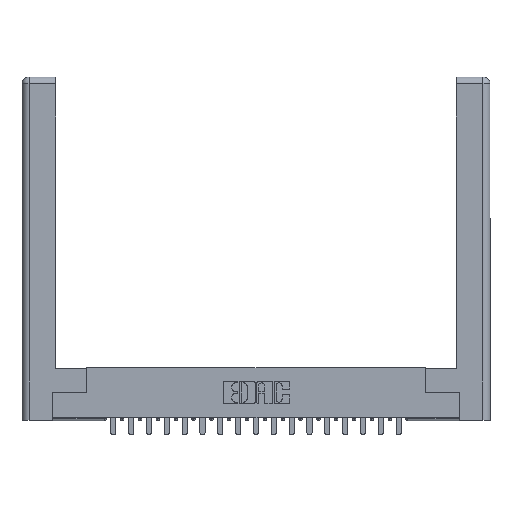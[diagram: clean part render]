
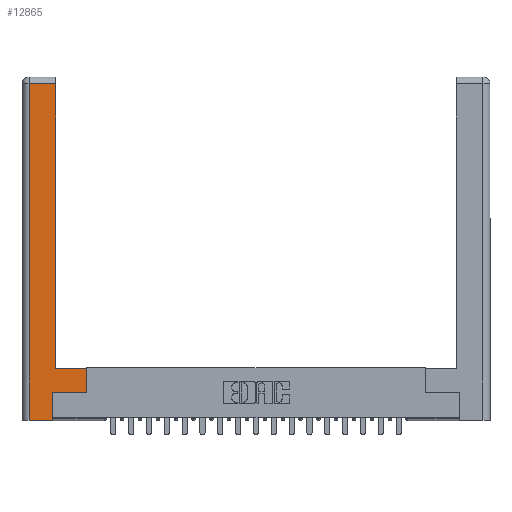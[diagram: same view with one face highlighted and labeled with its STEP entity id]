
A CAD part, top view. The second image highlights one B-rep face of the part: STEP entity #12865.
In plain terms, the highlighted planar face has unit normal (0, 0, 1).
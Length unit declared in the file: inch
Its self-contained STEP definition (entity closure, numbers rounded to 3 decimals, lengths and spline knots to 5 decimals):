
#217 = VECTOR ( 'NONE', #2579, 39.37008 ) ;
#251 = VERTEX_POINT ( 'NONE', #19789 ) ;
#571 = CARTESIAN_POINT ( 'NONE',  ( 0.295, 0.45, 0. ) ) ;
#2059 = EDGE_CURVE ( 'NONE', #21015, #13240, #12408, .T. ) ;
#2579 = DIRECTION ( 'NONE',  ( 1., 0., 0. ) ) ;
#3246 = DIRECTION ( 'NONE',  ( -1., 0., 0. ) ) ;
#3334 = PLANE ( 'NONE',  #18562 ) ;
#3410 = VECTOR ( 'NONE', #20492, 39.37008 ) ;
#3704 = ORIENTED_EDGE ( 'NONE', *, *, #23173, .T. ) ;
#3759 = DIRECTION ( 'NONE',  ( 0., -1., 0. ) ) ;
#4074 = CARTESIAN_POINT ( 'NONE',  ( 0.0615, 0., 0. ) ) ;
#4550 = ORIENTED_EDGE ( 'NONE', *, *, #2059, .T. ) ;
#4718 = CARTESIAN_POINT ( 'NONE',  ( 0.265, 0.245, 0. ) ) ;
#5852 = LINE ( 'NONE', #7973, #15176 ) ;
#6059 = DIRECTION ( 'NONE',  ( -1., 0., 0. ) ) ;
#6179 = CARTESIAN_POINT ( 'NONE',  ( 0.565, 0.45, 0. ) ) ;
#6319 = DIRECTION ( 'NONE',  ( 0., 1., 0. ) ) ;
#6332 = DIRECTION ( 'NONE',  ( -1., 0., 0. ) ) ;
#6421 = FACE_OUTER_BOUND ( 'NONE', #18535, .T. ) ;
#7001 = VERTEX_POINT ( 'NONE', #9324 ) ;
#7973 = CARTESIAN_POINT ( 'NONE',  ( 0.295, 0.45, 0. ) ) ;
#8054 = EDGE_CURVE ( 'NONE', #251, #20877, #14754, .T. ) ;
#8365 = ORIENTED_EDGE ( 'NONE', *, *, #20560, .T. ) ;
#8759 = CARTESIAN_POINT ( 'NONE',  ( 0., 0., 0. ) ) ;
#8888 = CARTESIAN_POINT ( 'NONE',  ( 0.565, 0.245, 0. ) ) ;
#9078 = DIRECTION ( 'NONE',  ( 0., 1., 0. ) ) ;
#9324 = CARTESIAN_POINT ( 'NONE',  ( 0.265, 0., 0. ) ) ;
#9907 = LINE ( 'NONE', #23638, #19163 ) ;
#9926 = EDGE_CURVE ( 'NONE', #14720, #12244, #15286, .T. ) ;
#10376 = ORIENTED_EDGE ( 'NONE', *, *, #16593, .T. ) ;
#10413 = ORIENTED_EDGE ( 'NONE', *, *, #12035, .T. ) ;
#10781 = DIRECTION ( 'NONE',  ( 1., 0., 0. ) ) ;
#12035 = EDGE_CURVE ( 'NONE', #12323, #251, #16365, .T. ) ;
#12057 = CARTESIAN_POINT ( 'NONE',  ( 0.0615, 0., 0. ) ) ;
#12240 = ORIENTED_EDGE ( 'NONE', *, *, #18211, .T. ) ;
#12244 = VERTEX_POINT ( 'NONE', #12057 ) ;
#12323 = VERTEX_POINT ( 'NONE', #4718 ) ;
#12408 = LINE ( 'NONE', #17141, #20802 ) ;
#12722 = CARTESIAN_POINT ( 'NONE',  ( 0.0615, 2.94, 0. ) ) ;
#12865 = ADVANCED_FACE ( 'NONE', ( #6421 ), #3334, .F. ) ;
#12906 = VECTOR ( 'NONE', #3759, 39.37008 ) ;
#13240 = VERTEX_POINT ( 'NONE', #16415 ) ;
#14352 = DIRECTION ( 'NONE',  ( 0., 0., -1. ) ) ;
#14720 = VERTEX_POINT ( 'NONE', #12722 ) ;
#14754 = LINE ( 'NONE', #20574, #3410 ) ;
#15176 = VECTOR ( 'NONE', #6332, 39.37008 ) ;
#15286 = LINE ( 'NONE', #4074, #12906 ) ;
#16306 = ORIENTED_EDGE ( 'NONE', *, *, #8054, .T. ) ;
#16365 = LINE ( 'NONE', #8888, #20684 ) ;
#16415 = CARTESIAN_POINT ( 'NONE',  ( 0.295, 2.94, 0. ) ) ;
#16593 = EDGE_CURVE ( 'NONE', #12244, #7001, #18201, .T. ) ;
#17141 = CARTESIAN_POINT ( 'NONE',  ( 0.295, 3., 0. ) ) ;
#18081 = ORIENTED_EDGE ( 'NONE', *, *, #9926, .T. ) ;
#18201 = LINE ( 'NONE', #20940, #217 ) ;
#18211 = EDGE_CURVE ( 'NONE', #7001, #12323, #9907, .T. ) ;
#18535 = EDGE_LOOP ( 'NONE', ( #4550, #8365, #18081, #10376, #12240, #10413, #16306, #3704 ) ) ;
#18562 = AXIS2_PLACEMENT_3D ( 'NONE', #8759, #14352, #3246 ) ;
#18880 = CARTESIAN_POINT ( 'NONE',  ( 0.0615, 2.94, 0. ) ) ;
#19163 = VECTOR ( 'NONE', #9078, 39.37008 ) ;
#19789 = CARTESIAN_POINT ( 'NONE',  ( 0.565, 0.245, 0. ) ) ;
#20492 = DIRECTION ( 'NONE',  ( 0., 1., 0. ) ) ;
#20560 = EDGE_CURVE ( 'NONE', #13240, #14720, #22535, .T. ) ;
#20574 = CARTESIAN_POINT ( 'NONE',  ( 0.565, 0.45, 0. ) ) ;
#20684 = VECTOR ( 'NONE', #10781, 39.37008 ) ;
#20802 = VECTOR ( 'NONE', #6319, 39.37008 ) ;
#20877 = VERTEX_POINT ( 'NONE', #6179 ) ;
#20940 = CARTESIAN_POINT ( 'NONE',  ( 0.265, 0., 0. ) ) ;
#21015 = VERTEX_POINT ( 'NONE', #571 ) ;
#22535 = LINE ( 'NONE', #18880, #23951 ) ;
#23173 = EDGE_CURVE ( 'NONE', #20877, #21015, #5852, .T. ) ;
#23638 = CARTESIAN_POINT ( 'NONE',  ( 0.265, 0.245, 0. ) ) ;
#23951 = VECTOR ( 'NONE', #6059, 39.37008 ) ;
